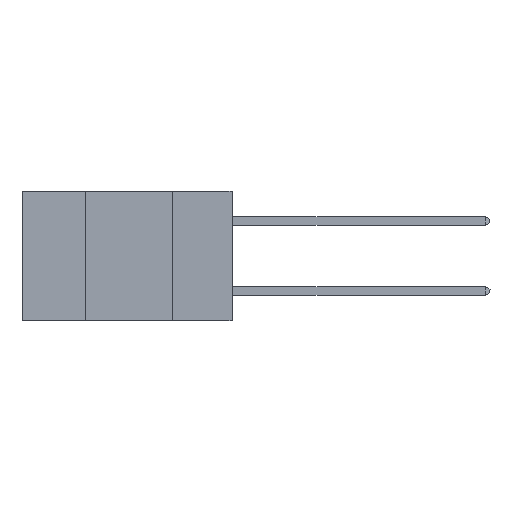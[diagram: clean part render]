
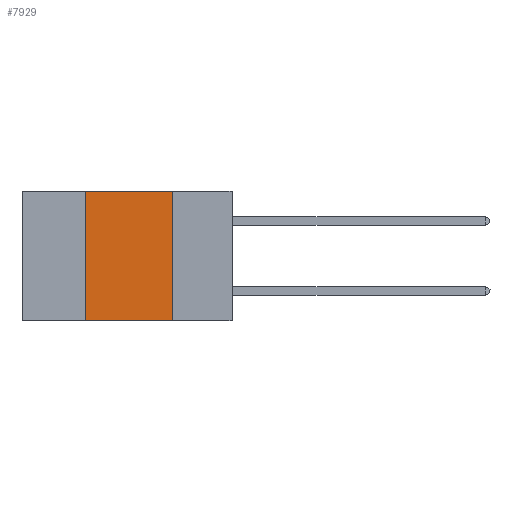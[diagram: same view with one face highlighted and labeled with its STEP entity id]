
A CAD part, left-side view. The second image highlights one B-rep face of the part: STEP entity #7929.
In plain terms, the highlighted planar face has unit normal (-1, 0, 0).
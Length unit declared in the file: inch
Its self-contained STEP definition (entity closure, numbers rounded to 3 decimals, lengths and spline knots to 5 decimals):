
#35 = EDGE_LOOP ( 'NONE', ( #12071, #6522, #12931, #13063 ) ) ;
#347 = DIRECTION ( 'NONE',  ( 0., 0., -1. ) ) ;
#532 = DIRECTION ( 'NONE',  ( 1., 0., 0. ) ) ;
#1120 = LINE ( 'NONE', #7407, #2892 ) ;
#1134 = EDGE_CURVE ( 'NONE', #8744, #3597, #1120, .T. ) ;
#1529 = VERTEX_POINT ( 'NONE', #11582 ) ;
#2414 = CARTESIAN_POINT ( 'NONE',  ( 0., 0.17, 0. ) ) ;
#2793 = VECTOR ( 'NONE', #347, 39.37008 ) ;
#2892 = VECTOR ( 'NONE', #6289, 39.37008 ) ;
#3110 = CARTESIAN_POINT ( 'NONE',  ( 0., 0.42, 0. ) ) ;
#3139 = VERTEX_POINT ( 'NONE', #7212 ) ;
#3597 = VERTEX_POINT ( 'NONE', #12309 ) ;
#3905 = CARTESIAN_POINT ( 'NONE',  ( 0., 0.6, 0. ) ) ;
#4621 = LINE ( 'NONE', #3905, #9071 ) ;
#5480 = EDGE_CURVE ( 'NONE', #8744, #1529, #8468, .T. ) ;
#6289 = DIRECTION ( 'NONE',  ( 0., -1., 0. ) ) ;
#6522 = ORIENTED_EDGE ( 'NONE', *, *, #13205, .F. ) ;
#7212 = CARTESIAN_POINT ( 'NONE',  ( 0., 0.17, 0. ) ) ;
#7348 = FACE_OUTER_BOUND ( 'NONE', #35, .T. ) ;
#7407 = CARTESIAN_POINT ( 'NONE',  ( 0., 0.6, -0.37 ) ) ;
#7609 = CARTESIAN_POINT ( 'NONE',  ( 0., 0.6, 0. ) ) ;
#7929 = ADVANCED_FACE ( 'NONE', ( #7348 ), #9814, .F. ) ;
#8003 = EDGE_CURVE ( 'NONE', #3139, #3597, #8635, .T. ) ;
#8468 = LINE ( 'NONE', #3110, #9302 ) ;
#8550 = DIRECTION ( 'NONE',  ( 0., 0., 1. ) ) ;
#8635 = LINE ( 'NONE', #2414, #2793 ) ;
#8744 = VERTEX_POINT ( 'NONE', #11390 ) ;
#8940 = AXIS2_PLACEMENT_3D ( 'NONE', #7609, #532, #9776 ) ;
#9071 = VECTOR ( 'NONE', #11633, 39.37008 ) ;
#9302 = VECTOR ( 'NONE', #8550, 39.37008 ) ;
#9776 = DIRECTION ( 'NONE',  ( 0., 0., -1. ) ) ;
#9814 = PLANE ( 'NONE',  #8940 ) ;
#11390 = CARTESIAN_POINT ( 'NONE',  ( 0., 0.42, -0.37 ) ) ;
#11582 = CARTESIAN_POINT ( 'NONE',  ( 0., 0.42, 0. ) ) ;
#11633 = DIRECTION ( 'NONE',  ( 0., -1., 0. ) ) ;
#12071 = ORIENTED_EDGE ( 'NONE', *, *, #8003, .F. ) ;
#12309 = CARTESIAN_POINT ( 'NONE',  ( 0., 0.17, -0.37 ) ) ;
#12931 = ORIENTED_EDGE ( 'NONE', *, *, #5480, .F. ) ;
#13063 = ORIENTED_EDGE ( 'NONE', *, *, #1134, .T. ) ;
#13205 = EDGE_CURVE ( 'NONE', #1529, #3139, #4621, .T. ) ;
